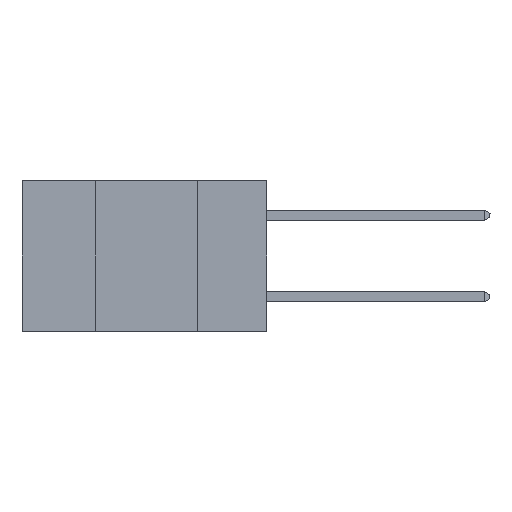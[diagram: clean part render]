
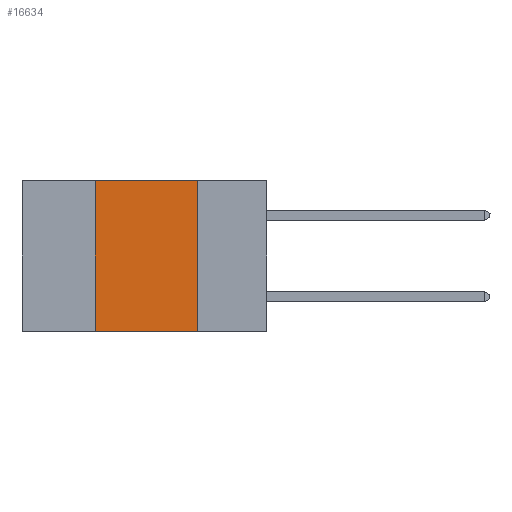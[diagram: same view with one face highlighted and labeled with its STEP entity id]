
A CAD part, left-side view. The second image highlights one B-rep face of the part: STEP entity #16634.
In plain terms, the highlighted planar face has unit normal (-1, 0, 0).
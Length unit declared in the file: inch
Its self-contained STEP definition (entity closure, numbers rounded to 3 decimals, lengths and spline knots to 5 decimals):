
#161 = FACE_OUTER_BOUND ( 'NONE', #2018, .T. ) ;
#377 = DIRECTION ( 'NONE',  ( 0., -1., 0. ) ) ;
#562 = ORIENTED_EDGE ( 'NONE', *, *, #16923, .T. ) ;
#712 = PLANE ( 'NONE',  #5729 ) ;
#2018 = EDGE_LOOP ( 'NONE', ( #17669, #9732, #11135, #562 ) ) ;
#3185 = LINE ( 'NONE', #9122, #9800 ) ;
#3334 = CARTESIAN_POINT ( 'NONE',  ( 0., 0.42, 0. ) ) ;
#3996 = VERTEX_POINT ( 'NONE', #14810 ) ;
#4304 = LINE ( 'NONE', #11929, #4420 ) ;
#4420 = VECTOR ( 'NONE', #19134, 39.37008 ) ;
#4573 = EDGE_CURVE ( 'NONE', #5265, #19157, #4810, .T. ) ;
#4810 = LINE ( 'NONE', #3334, #9260 ) ;
#5079 = DIRECTION ( 'NONE',  ( 0., 0., -1. ) ) ;
#5129 = VECTOR ( 'NONE', #8376, 39.37008 ) ;
#5265 = VERTEX_POINT ( 'NONE', #8653 ) ;
#5729 = AXIS2_PLACEMENT_3D ( 'NONE', #11947, #16990, #5079 ) ;
#8376 = DIRECTION ( 'NONE',  ( 0., -1., 0. ) ) ;
#8569 = CARTESIAN_POINT ( 'NONE',  ( 0., 0.6, -0.37 ) ) ;
#8653 = CARTESIAN_POINT ( 'NONE',  ( 0., 0.42, -0.37 ) ) ;
#9122 = CARTESIAN_POINT ( 'NONE',  ( 0., 0.6, 0. ) ) ;
#9193 = CARTESIAN_POINT ( 'NONE',  ( 0., 0.17, -0.37 ) ) ;
#9260 = VECTOR ( 'NONE', #16911, 39.37008 ) ;
#9732 = ORIENTED_EDGE ( 'NONE', *, *, #17631, .F. ) ;
#9800 = VECTOR ( 'NONE', #377, 39.37008 ) ;
#11135 = ORIENTED_EDGE ( 'NONE', *, *, #4573, .F. ) ;
#11378 = CARTESIAN_POINT ( 'NONE',  ( 0., 0.42, 0. ) ) ;
#11929 = CARTESIAN_POINT ( 'NONE',  ( 0., 0.17, 0. ) ) ;
#11947 = CARTESIAN_POINT ( 'NONE',  ( 0., 0.6, 0. ) ) ;
#13818 = EDGE_CURVE ( 'NONE', #3996, #18140, #4304, .T. ) ;
#14810 = CARTESIAN_POINT ( 'NONE',  ( 0., 0.17, 0. ) ) ;
#16011 = LINE ( 'NONE', #8569, #5129 ) ;
#16634 = ADVANCED_FACE ( 'NONE', ( #161 ), #712, .F. ) ;
#16911 = DIRECTION ( 'NONE',  ( 0., 0., 1. ) ) ;
#16923 = EDGE_CURVE ( 'NONE', #5265, #18140, #16011, .T. ) ;
#16990 = DIRECTION ( 'NONE',  ( 1., 0., 0. ) ) ;
#17631 = EDGE_CURVE ( 'NONE', #19157, #3996, #3185, .T. ) ;
#17669 = ORIENTED_EDGE ( 'NONE', *, *, #13818, .F. ) ;
#18140 = VERTEX_POINT ( 'NONE', #9193 ) ;
#19134 = DIRECTION ( 'NONE',  ( 0., 0., -1. ) ) ;
#19157 = VERTEX_POINT ( 'NONE', #11378 ) ;
